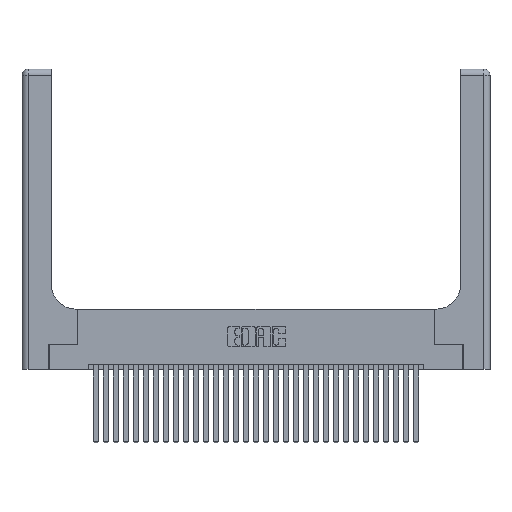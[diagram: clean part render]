
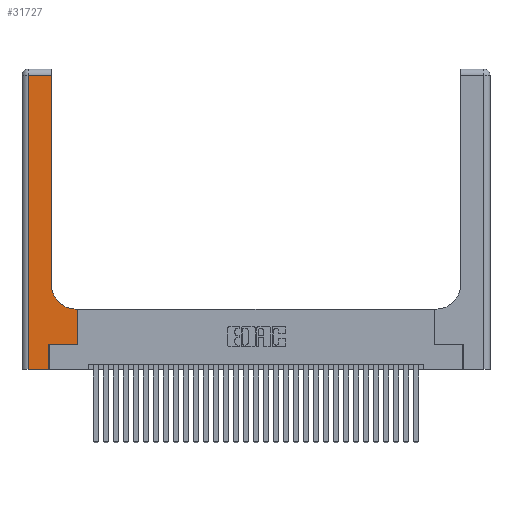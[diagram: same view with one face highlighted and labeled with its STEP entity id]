
A CAD part, top view. The second image highlights one B-rep face of the part: STEP entity #31727.
In plain terms, the highlighted planar face has unit normal (0, 0, 1).
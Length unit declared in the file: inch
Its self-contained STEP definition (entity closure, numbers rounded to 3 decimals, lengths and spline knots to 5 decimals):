
#206 = EDGE_CURVE ( 'NONE', #10297, #12538, #26721, .T. ) ;
#400 = CARTESIAN_POINT ( 'NONE',  ( 0.5585, 0.25, 0.37 ) ) ;
#749 = EDGE_CURVE ( 'NONE', #27900, #20281, #26326, .T. ) ;
#844 = EDGE_CURVE ( 'NONE', #27628, #13737, #23973, .T. ) ;
#1440 = VECTOR ( 'NONE', #29531, 39.37008 ) ;
#1660 = EDGE_CURVE ( 'NONE', #13737, #27900, #6893, .T. ) ;
#1768 = VERTEX_POINT ( 'NONE', #1944 ) ;
#1815 = CARTESIAN_POINT ( 'NONE',  ( 0.269, 0.25, 0.37 ) ) ;
#1869 = VECTOR ( 'NONE', #26845, 39.37008 ) ;
#1944 = CARTESIAN_POINT ( 'NONE',  ( 0.2915, 2.94, 0.37 ) ) ;
#2908 = CARTESIAN_POINT ( 'NONE',  ( 0.269, 0., 0.37 ) ) ;
#2919 = LINE ( 'NONE', #400, #14567 ) ;
#3069 = CARTESIAN_POINT ( 'NONE',  ( 0.06, 2.94, 0.37 ) ) ;
#3082 = CARTESIAN_POINT ( 'NONE',  ( 0., 2.94, 0.37 ) ) ;
#4038 = DIRECTION ( 'NONE',  ( 0., 1., 0. ) ) ;
#4183 = VECTOR ( 'NONE', #5279, 39.37008 ) ;
#4811 = CARTESIAN_POINT ( 'NONE',  ( 0.5585, 0.6, 0.37 ) ) ;
#5155 = VERTEX_POINT ( 'NONE', #4811 ) ;
#5279 = DIRECTION ( 'NONE',  ( 1., 0., 0. ) ) ;
#6628 = VERTEX_POINT ( 'NONE', #3069 ) ;
#6893 = LINE ( 'NONE', #19157, #7660 ) ;
#7423 = EDGE_CURVE ( 'NONE', #5155, #10297, #17620, .T. ) ;
#7660 = VECTOR ( 'NONE', #13516, 39.37008 ) ;
#8224 = ORIENTED_EDGE ( 'NONE', *, *, #12338, .T. ) ;
#8247 = DIRECTION ( 'NONE',  ( 0., 1., 0. ) ) ;
#8691 = ORIENTED_EDGE ( 'NONE', *, *, #17168, .T. ) ;
#9725 = CARTESIAN_POINT ( 'NONE',  ( 0.06, 3., 0.37 ) ) ;
#10297 = VERTEX_POINT ( 'NONE', #20716 ) ;
#10681 = VECTOR ( 'NONE', #4038, 39.37008 ) ;
#11138 = EDGE_LOOP ( 'NONE', ( #15025, #8691, #8224, #23249, #11716, #25107, #23991, #22688, #12175 ) ) ;
#11177 = FACE_OUTER_BOUND ( 'NONE', #11138, .T. ) ;
#11716 = ORIENTED_EDGE ( 'NONE', *, *, #1660, .T. ) ;
#12175 = ORIENTED_EDGE ( 'NONE', *, *, #206, .T. ) ;
#12338 = EDGE_CURVE ( 'NONE', #6628, #27628, #13107, .T. ) ;
#12538 = VERTEX_POINT ( 'NONE', #22275 ) ;
#12742 = DIRECTION ( 'NONE',  ( -1., 0., 0. ) ) ;
#12840 = PLANE ( 'NONE',  #23688 ) ;
#13060 = DIRECTION ( 'NONE',  ( -1., 0., 0. ) ) ;
#13107 = LINE ( 'NONE', #9725, #1440 ) ;
#13442 = DIRECTION ( 'NONE',  ( 0., 0., -1. ) ) ;
#13516 = DIRECTION ( 'NONE',  ( 0., 1., 0. ) ) ;
#13737 = VERTEX_POINT ( 'NONE', #2908 ) ;
#14567 = VECTOR ( 'NONE', #8247, 39.37008 ) ;
#15025 = ORIENTED_EDGE ( 'NONE', *, *, #15759, .T. ) ;
#15345 = DIRECTION ( 'NONE',  ( 0., 0., -1. ) ) ;
#15759 = EDGE_CURVE ( 'NONE', #12538, #1768, #23084, .T. ) ;
#16158 = CARTESIAN_POINT ( 'NONE',  ( 0.5415, 0.85, 0.37 ) ) ;
#17168 = EDGE_CURVE ( 'NONE', #1768, #6628, #28794, .T. ) ;
#17580 = CARTESIAN_POINT ( 'NONE',  ( 0.269, 0.25, 0.37 ) ) ;
#17620 = LINE ( 'NONE', #18892, #27295 ) ;
#18758 = DIRECTION ( 'NONE',  ( 1., 0., 0. ) ) ;
#18892 = CARTESIAN_POINT ( 'NONE',  ( 0.2915, 0.6, 0.37 ) ) ;
#19157 = CARTESIAN_POINT ( 'NONE',  ( 0.269, 0., 0.37 ) ) ;
#20281 = VERTEX_POINT ( 'NONE', #23119 ) ;
#20716 = CARTESIAN_POINT ( 'NONE',  ( 0.5415, 0.6, 0.37 ) ) ;
#21377 = DIRECTION ( 'NONE',  ( -1., 0., 0. ) ) ;
#21751 = EDGE_CURVE ( 'NONE', #20281, #5155, #2919, .T. ) ;
#21818 = VECTOR ( 'NONE', #13060, 39.37008 ) ;
#22275 = CARTESIAN_POINT ( 'NONE',  ( 0.2915, 0.85, 0.37 ) ) ;
#22688 = ORIENTED_EDGE ( 'NONE', *, *, #7423, .T. ) ;
#23084 = LINE ( 'NONE', #31576, #10681 ) ;
#23119 = CARTESIAN_POINT ( 'NONE',  ( 0.5585, 0.25, 0.37 ) ) ;
#23249 = ORIENTED_EDGE ( 'NONE', *, *, #844, .T. ) ;
#23688 = AXIS2_PLACEMENT_3D ( 'NONE', #27788, #15345, #12742 ) ;
#23973 = LINE ( 'NONE', #29667, #4183 ) ;
#23989 = CARTESIAN_POINT ( 'NONE',  ( 0.06, 0., 0.37 ) ) ;
#23991 = ORIENTED_EDGE ( 'NONE', *, *, #21751, .T. ) ;
#25107 = ORIENTED_EDGE ( 'NONE', *, *, #749, .T. ) ;
#26326 = LINE ( 'NONE', #1815, #1869 ) ;
#26721 = CIRCLE ( 'NONE', #27659, 0.25 ) ;
#26845 = DIRECTION ( 'NONE',  ( 1., 0., 0. ) ) ;
#27295 = VECTOR ( 'NONE', #21377, 39.37008 ) ;
#27628 = VERTEX_POINT ( 'NONE', #23989 ) ;
#27659 = AXIS2_PLACEMENT_3D ( 'NONE', #16158, #13442, #18758 ) ;
#27788 = CARTESIAN_POINT ( 'NONE',  ( 0., 3., 0.37 ) ) ;
#27900 = VERTEX_POINT ( 'NONE', #17580 ) ;
#28794 = LINE ( 'NONE', #3082, #21818 ) ;
#29531 = DIRECTION ( 'NONE',  ( 0., -1., 0. ) ) ;
#29667 = CARTESIAN_POINT ( 'NONE',  ( 0., 0., 0.37 ) ) ;
#31576 = CARTESIAN_POINT ( 'NONE',  ( 0.2915, 3., 0.37 ) ) ;
#31727 = ADVANCED_FACE ( 'NONE', ( #11177 ), #12840, .F. ) ;
